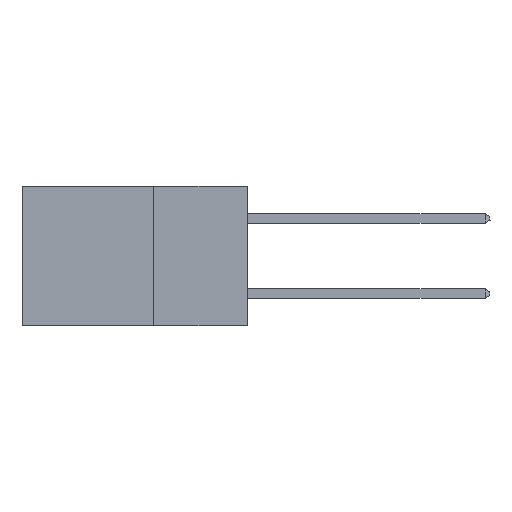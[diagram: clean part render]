
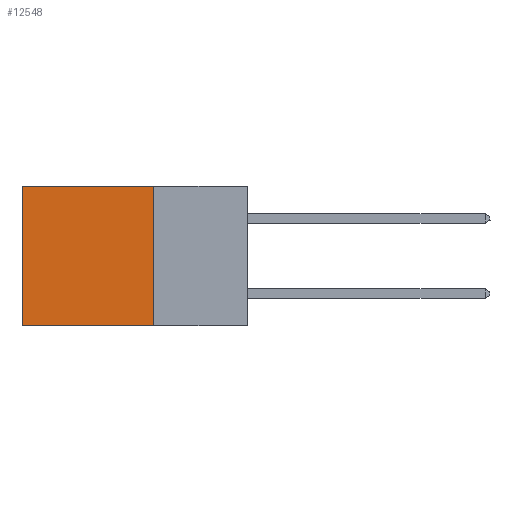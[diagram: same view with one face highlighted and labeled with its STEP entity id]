
A CAD part, left-side view. The second image highlights one B-rep face of the part: STEP entity #12548.
In plain terms, the highlighted planar face has unit normal (-1, 0, 0).
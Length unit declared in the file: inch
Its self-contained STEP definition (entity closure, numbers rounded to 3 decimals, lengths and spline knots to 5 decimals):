
#2 = VERTEX_POINT ( 'NONE', #4873 ) ;
#232 = DIRECTION ( 'NONE',  ( 0., 0., -1. ) ) ;
#1132 = EDGE_LOOP ( 'NONE', ( #28816, #23603, #33702, #2913 ) ) ;
#2524 = DIRECTION ( 'NONE',  ( 1., 0., 0. ) ) ;
#2666 = CARTESIAN_POINT ( 'NONE',  ( 0.298, 0.6, 0. ) ) ;
#2913 = ORIENTED_EDGE ( 'NONE', *, *, #24135, .T. ) ;
#3505 = CARTESIAN_POINT ( 'NONE',  ( 0.298, 0.25, -0.37 ) ) ;
#4873 = CARTESIAN_POINT ( 'NONE',  ( 0.298, 0.25, -0.37 ) ) ;
#4976 = VERTEX_POINT ( 'NONE', #19975 ) ;
#5196 = DIRECTION ( 'NONE',  ( 0., 0., -1. ) ) ;
#5212 = FACE_OUTER_BOUND ( 'NONE', #1132, .T. ) ;
#5848 = LINE ( 'NONE', #10844, #16266 ) ;
#8862 = DIRECTION ( 'NONE',  ( 0., 1., 0. ) ) ;
#10844 = CARTESIAN_POINT ( 'NONE',  ( 0.298, 0.25, 0. ) ) ;
#12548 = ADVANCED_FACE ( 'NONE', ( #5212 ), #18327, .F. ) ;
#14377 = VECTOR ( 'NONE', #30701, 39.37008 ) ;
#14956 = LINE ( 'NONE', #3505, #28608 ) ;
#16106 = CARTESIAN_POINT ( 'NONE',  ( 0.298, 0.25, 0. ) ) ;
#16266 = VECTOR ( 'NONE', #24165, 39.37008 ) ;
#18327 = PLANE ( 'NONE',  #20877 ) ;
#18773 = VERTEX_POINT ( 'NONE', #33719 ) ;
#19975 = CARTESIAN_POINT ( 'NONE',  ( 0.298, 0.25, 0. ) ) ;
#20482 = CARTESIAN_POINT ( 'NONE',  ( 0.298, 0.6, 0. ) ) ;
#20877 = AXIS2_PLACEMENT_3D ( 'NONE', #16106, #2524, #232 ) ;
#21602 = EDGE_CURVE ( 'NONE', #32761, #18773, #33526, .T. ) ;
#23603 = ORIENTED_EDGE ( 'NONE', *, *, #26617, .F. ) ;
#24135 = EDGE_CURVE ( 'NONE', #4976, #32761, #5848, .T. ) ;
#24165 = DIRECTION ( 'NONE',  ( 0., 1., 0. ) ) ;
#26617 = EDGE_CURVE ( 'NONE', #2, #18773, #14956, .T. ) ;
#27647 = LINE ( 'NONE', #28012, #14377 ) ;
#28012 = CARTESIAN_POINT ( 'NONE',  ( 0.298, 0.25, 0. ) ) ;
#28608 = VECTOR ( 'NONE', #8862, 39.37008 ) ;
#28816 = ORIENTED_EDGE ( 'NONE', *, *, #21602, .T. ) ;
#30120 = EDGE_CURVE ( 'NONE', #4976, #2, #27647, .T. ) ;
#30701 = DIRECTION ( 'NONE',  ( 0., 0., -1. ) ) ;
#31010 = VECTOR ( 'NONE', #5196, 39.37008 ) ;
#32761 = VERTEX_POINT ( 'NONE', #20482 ) ;
#33526 = LINE ( 'NONE', #2666, #31010 ) ;
#33702 = ORIENTED_EDGE ( 'NONE', *, *, #30120, .F. ) ;
#33719 = CARTESIAN_POINT ( 'NONE',  ( 0.298, 0.6, -0.37 ) ) ;
